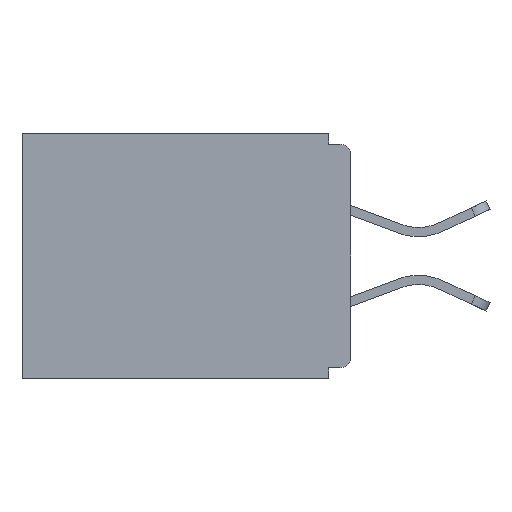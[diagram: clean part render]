
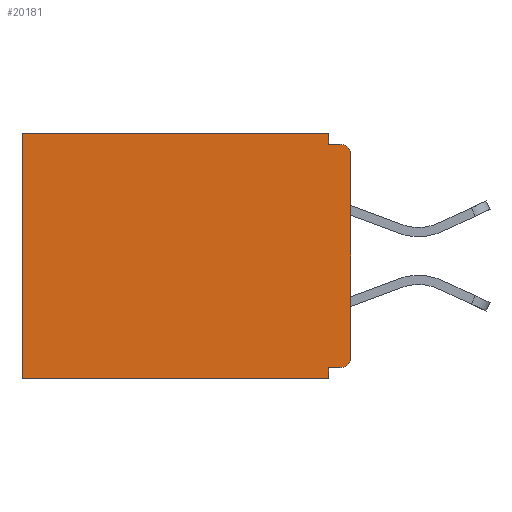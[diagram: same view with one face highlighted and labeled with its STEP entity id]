
A CAD part, left-side view. The second image highlights one B-rep face of the part: STEP entity #20181.
In plain terms, the highlighted planar face has unit normal (-1, 0, 0).
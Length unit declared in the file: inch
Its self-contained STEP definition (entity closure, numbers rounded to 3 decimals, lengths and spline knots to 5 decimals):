
#101 = VERTEX_POINT ( 'NONE', #1724 ) ;
#299 = EDGE_CURVE ( 'NONE', #20539, #27028, #18737, .T. ) ;
#395 = ORIENTED_EDGE ( 'NONE', *, *, #1321, .F. ) ;
#941 = VECTOR ( 'NONE', #19018, 39.37008 ) ;
#1116 = CARTESIAN_POINT ( 'NONE',  ( 0.298, 0., 0. ) ) ;
#1321 = EDGE_CURVE ( 'NONE', #30552, #28183, #11940, .T. ) ;
#1392 = CIRCLE ( 'NONE', #14127, 0.015 ) ;
#1559 = VERTEX_POINT ( 'NONE', #1692 ) ;
#1692 = CARTESIAN_POINT ( 'NONE',  ( 0.298, 0.46, -0.343 ) ) ;
#1724 = CARTESIAN_POINT ( 'NONE',  ( 0.298, 0., -0.03 ) ) ;
#1733 = DIRECTION ( 'NONE',  ( 0., -1., 0. ) ) ;
#1991 = EDGE_CURVE ( 'NONE', #18680, #14624, #29134, .T. ) ;
#2220 = LINE ( 'NONE', #19084, #30301 ) ;
#2828 = CARTESIAN_POINT ( 'NONE',  ( 0.298, 0.015, -0.328 ) ) ;
#2983 = ORIENTED_EDGE ( 'NONE', *, *, #4835, .F. ) ;
#3701 = CARTESIAN_POINT ( 'NONE',  ( 0.298, 0.031, -0.343 ) ) ;
#4240 = FACE_OUTER_BOUND ( 'NONE', #14847, .T. ) ;
#4835 = EDGE_CURVE ( 'NONE', #101, #24516, #28238, .T. ) ;
#5032 = CARTESIAN_POINT ( 'NONE',  ( 0.298, 0.015, -0.313 ) ) ;
#5288 = VECTOR ( 'NONE', #27258, 39.37008 ) ;
#5391 = EDGE_CURVE ( 'NONE', #20971, #24516, #28184, .T. ) ;
#5752 = LINE ( 'NONE', #10598, #15482 ) ;
#5887 = EDGE_CURVE ( 'NONE', #20539, #30552, #27773, .T. ) ;
#5898 = ORIENTED_EDGE ( 'NONE', *, *, #5391, .T. ) ;
#6015 = CARTESIAN_POINT ( 'NONE',  ( 0.298, 0.015, -0.03 ) ) ;
#7240 = DIRECTION ( 'NONE',  ( -1., 0., 0. ) ) ;
#8023 = DIRECTION ( 'NONE',  ( 0., 1., 0. ) ) ;
#8240 = ORIENTED_EDGE ( 'NONE', *, *, #22168, .F. ) ;
#8956 = DIRECTION ( 'NONE',  ( 0., 0., -1. ) ) ;
#8964 = EDGE_CURVE ( 'NONE', #101, #28183, #1392, .T. ) ;
#9852 = DIRECTION ( 'NONE',  ( 1., 0., 0. ) ) ;
#9949 = PLANE ( 'NONE',  #20151 ) ;
#10429 = VECTOR ( 'NONE', #1733, 39.37008 ) ;
#10598 = CARTESIAN_POINT ( 'NONE',  ( 0.298, 0., -0.343 ) ) ;
#10861 = DIRECTION ( 'NONE',  ( 0., 0., -1. ) ) ;
#11026 = DIRECTION ( 'NONE',  ( 0., 1., 0. ) ) ;
#11066 = LINE ( 'NONE', #16581, #941 ) ;
#11413 = ORIENTED_EDGE ( 'NONE', *, *, #1991, .F. ) ;
#11698 = AXIS2_PLACEMENT_3D ( 'NONE', #5032, #7240, #26615 ) ;
#11940 = LINE ( 'NONE', #30292, #10429 ) ;
#12128 = VECTOR ( 'NONE', #19272, 39.37008 ) ;
#12374 = VECTOR ( 'NONE', #8023, 39.37008 ) ;
#14127 = AXIS2_PLACEMENT_3D ( 'NONE', #6015, #17838, #10861 ) ;
#14624 = VERTEX_POINT ( 'NONE', #22493 ) ;
#14847 = EDGE_LOOP ( 'NONE', ( #21167, #395, #16410, #25888, #26356, #21884, #11413, #8240, #5898, #2983 ) ) ;
#14923 = CARTESIAN_POINT ( 'NONE',  ( 0.298, 0., 0. ) ) ;
#15287 = CARTESIAN_POINT ( 'NONE',  ( 0.298, 0.031, 0. ) ) ;
#15482 = VECTOR ( 'NONE', #11026, 39.37008 ) ;
#16350 = VECTOR ( 'NONE', #8956, 39.37008 ) ;
#16410 = ORIENTED_EDGE ( 'NONE', *, *, #5887, .F. ) ;
#16581 = CARTESIAN_POINT ( 'NONE',  ( 0.298, 0.46, 0. ) ) ;
#16918 = CARTESIAN_POINT ( 'NONE',  ( 0.298, 0., -0.313 ) ) ;
#17838 = DIRECTION ( 'NONE',  ( -1., 0., 0. ) ) ;
#18594 = EDGE_CURVE ( 'NONE', #27028, #1559, #11066, .T. ) ;
#18680 = VERTEX_POINT ( 'NONE', #18995 ) ;
#18737 = LINE ( 'NONE', #1116, #12374 ) ;
#18995 = CARTESIAN_POINT ( 'NONE',  ( 0.298, 0.031, -0.328 ) ) ;
#19018 = DIRECTION ( 'NONE',  ( 0., 0., -1. ) ) ;
#19084 = CARTESIAN_POINT ( 'NONE',  ( 0.298, 0., -0.328 ) ) ;
#19272 = DIRECTION ( 'NONE',  ( 0., 0., -1. ) ) ;
#19463 = DIRECTION ( 'NONE',  ( 0., 0., -1. ) ) ;
#20151 = AXIS2_PLACEMENT_3D ( 'NONE', #14923, #9852, #19463 ) ;
#20181 = ADVANCED_FACE ( 'NONE', ( #4240 ), #9949, .F. ) ;
#20539 = VERTEX_POINT ( 'NONE', #15287 ) ;
#20889 = CARTESIAN_POINT ( 'NONE',  ( 0.298, 0.015, -0.015 ) ) ;
#20971 = VERTEX_POINT ( 'NONE', #2828 ) ;
#21167 = ORIENTED_EDGE ( 'NONE', *, *, #8964, .T. ) ;
#21281 = CARTESIAN_POINT ( 'NONE',  ( 0.298, 0.031, -0.343 ) ) ;
#21473 = CARTESIAN_POINT ( 'NONE',  ( 0.298, 0.46, 0. ) ) ;
#21884 = ORIENTED_EDGE ( 'NONE', *, *, #26808, .F. ) ;
#22168 = EDGE_CURVE ( 'NONE', #20971, #18680, #2220, .T. ) ;
#22493 = CARTESIAN_POINT ( 'NONE',  ( 0.298, 0.031, -0.343 ) ) ;
#23214 = CARTESIAN_POINT ( 'NONE',  ( 0.298, 0.031, -0.015 ) ) ;
#24516 = VERTEX_POINT ( 'NONE', #16918 ) ;
#25888 = ORIENTED_EDGE ( 'NONE', *, *, #299, .T. ) ;
#26356 = ORIENTED_EDGE ( 'NONE', *, *, #18594, .T. ) ;
#26615 = DIRECTION ( 'NONE',  ( 0., 0., -1. ) ) ;
#26808 = EDGE_CURVE ( 'NONE', #14624, #1559, #5752, .T. ) ;
#27028 = VERTEX_POINT ( 'NONE', #21473 ) ;
#27258 = DIRECTION ( 'NONE',  ( 0., 0., -1. ) ) ;
#27773 = LINE ( 'NONE', #3701, #5288 ) ;
#28183 = VERTEX_POINT ( 'NONE', #20889 ) ;
#28184 = CIRCLE ( 'NONE', #11698, 0.015 ) ;
#28238 = LINE ( 'NONE', #28614, #12128 ) ;
#28614 = CARTESIAN_POINT ( 'NONE',  ( 0.298, 0., 0. ) ) ;
#29134 = LINE ( 'NONE', #21281, #16350 ) ;
#30292 = CARTESIAN_POINT ( 'NONE',  ( 0.298, 0., -0.015 ) ) ;
#30301 = VECTOR ( 'NONE', #30789, 39.37008 ) ;
#30552 = VERTEX_POINT ( 'NONE', #23214 ) ;
#30789 = DIRECTION ( 'NONE',  ( 0., 1., 0. ) ) ;
